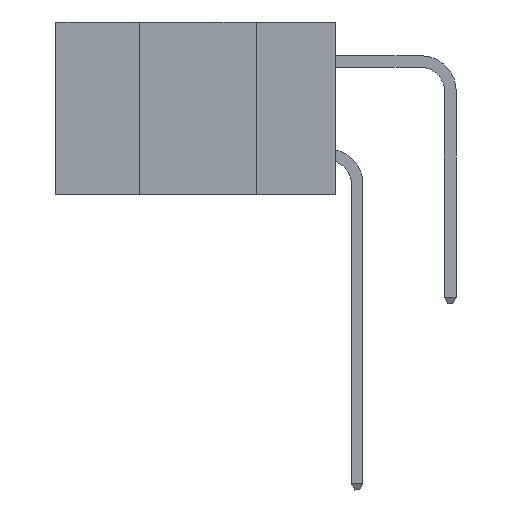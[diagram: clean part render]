
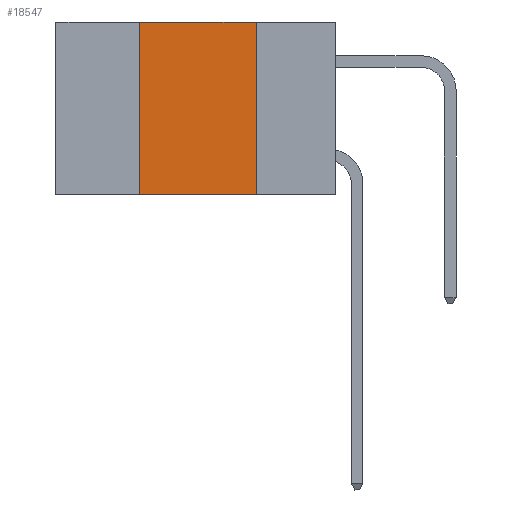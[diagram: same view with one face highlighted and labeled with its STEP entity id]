
A CAD part, left-side view. The second image highlights one B-rep face of the part: STEP entity #18547.
In plain terms, the highlighted planar face has unit normal (-1, 0, 0).
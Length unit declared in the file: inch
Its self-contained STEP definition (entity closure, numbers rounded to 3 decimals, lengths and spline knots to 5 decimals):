
#926 = VERTEX_POINT ( 'NONE', #37338 ) ;
#2358 = CARTESIAN_POINT ( 'NONE',  ( 0., 0.42, -0.37 ) ) ;
#2482 = CARTESIAN_POINT ( 'NONE',  ( 0., 0.17, 0. ) ) ;
#2871 = FACE_OUTER_BOUND ( 'NONE', #37920, .T. ) ;
#3469 = DIRECTION ( 'NONE',  ( 0., -1., 0. ) ) ;
#5236 = LINE ( 'NONE', #38111, #14504 ) ;
#5731 = DIRECTION ( 'NONE',  ( 0., 0., -1. ) ) ;
#6880 = VERTEX_POINT ( 'NONE', #8875 ) ;
#7334 = DIRECTION ( 'NONE',  ( 0., 0., 1. ) ) ;
#8807 = ORIENTED_EDGE ( 'NONE', *, *, #40165, .F. ) ;
#8875 = CARTESIAN_POINT ( 'NONE',  ( 0., 0.17, 0. ) ) ;
#9519 = CARTESIAN_POINT ( 'NONE',  ( 0., 0.17, -0.37 ) ) ;
#10539 = LINE ( 'NONE', #2482, #20872 ) ;
#12607 = DIRECTION ( 'NONE',  ( 1., 0., 0. ) ) ;
#14504 = VECTOR ( 'NONE', #3469, 39.37008 ) ;
#16223 = VERTEX_POINT ( 'NONE', #9519 ) ;
#16369 = CARTESIAN_POINT ( 'NONE',  ( 0., 0.6, 0. ) ) ;
#18547 = ADVANCED_FACE ( 'NONE', ( #2871 ), #36589, .F. ) ;
#19714 = LINE ( 'NONE', #31518, #34394 ) ;
#19932 = VERTEX_POINT ( 'NONE', #2358 ) ;
#20872 = VECTOR ( 'NONE', #40966, 39.37008 ) ;
#23313 = ORIENTED_EDGE ( 'NONE', *, *, #36074, .F. ) ;
#23819 = EDGE_CURVE ( 'NONE', #19932, #926, #19714, .T. ) ;
#24861 = AXIS2_PLACEMENT_3D ( 'NONE', #16369, #12607, #5731 ) ;
#25212 = EDGE_CURVE ( 'NONE', #19932, #16223, #36449, .T. ) ;
#29439 = CARTESIAN_POINT ( 'NONE',  ( 0., 0.6, -0.37 ) ) ;
#30510 = VECTOR ( 'NONE', #32451, 39.37008 ) ;
#31518 = CARTESIAN_POINT ( 'NONE',  ( 0., 0.42, 0. ) ) ;
#32451 = DIRECTION ( 'NONE',  ( 0., -1., 0. ) ) ;
#33443 = ORIENTED_EDGE ( 'NONE', *, *, #23819, .F. ) ;
#34394 = VECTOR ( 'NONE', #7334, 39.37008 ) ;
#36074 = EDGE_CURVE ( 'NONE', #6880, #16223, #10539, .T. ) ;
#36449 = LINE ( 'NONE', #29439, #30510 ) ;
#36589 = PLANE ( 'NONE',  #24861 ) ;
#37338 = CARTESIAN_POINT ( 'NONE',  ( 0., 0.42, 0. ) ) ;
#37920 = EDGE_LOOP ( 'NONE', ( #23313, #8807, #33443, #41195 ) ) ;
#38111 = CARTESIAN_POINT ( 'NONE',  ( 0., 0.6, 0. ) ) ;
#40165 = EDGE_CURVE ( 'NONE', #926, #6880, #5236, .T. ) ;
#40966 = DIRECTION ( 'NONE',  ( 0., 0., -1. ) ) ;
#41195 = ORIENTED_EDGE ( 'NONE', *, *, #25212, .T. ) ;
